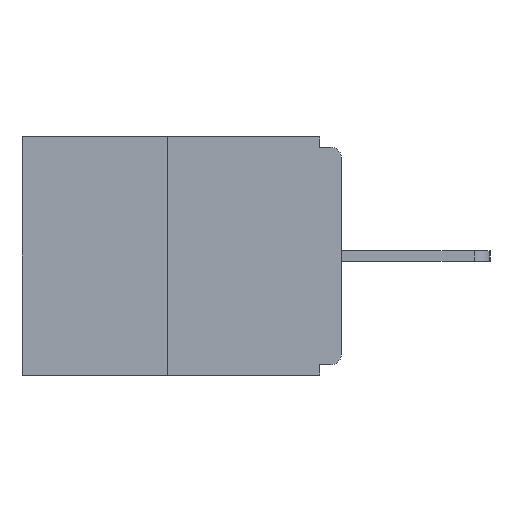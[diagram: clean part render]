
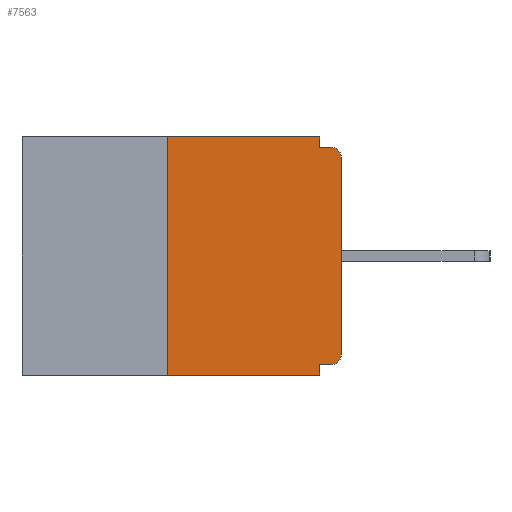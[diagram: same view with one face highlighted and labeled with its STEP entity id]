
A CAD part, left-side view. The second image highlights one B-rep face of the part: STEP entity #7563.
In plain terms, the highlighted planar face has unit normal (-1, 0, 0).
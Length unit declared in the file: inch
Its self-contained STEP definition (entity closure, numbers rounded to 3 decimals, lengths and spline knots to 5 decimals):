
#67 = ORIENTED_EDGE ( 'NONE', *, *, #9139, .T. ) ;
#259 = CARTESIAN_POINT ( 'NONE',  ( 0., 0.46, 0. ) ) ;
#504 = CARTESIAN_POINT ( 'NONE',  ( 0., 0.031, -0.343 ) ) ;
#523 = DIRECTION ( 'NONE',  ( 0., 0., -1. ) ) ;
#675 = ORIENTED_EDGE ( 'NONE', *, *, #9671, .F. ) ;
#726 = PLANE ( 'NONE',  #10815 ) ;
#740 = VECTOR ( 'NONE', #11413, 39.37008 ) ;
#1176 = LINE ( 'NONE', #8990, #740 ) ;
#1315 = DIRECTION ( 'NONE',  ( 0., 0., 1. ) ) ;
#1775 = EDGE_CURVE ( 'NONE', #8409, #5490, #1176, .T. ) ;
#1778 = CARTESIAN_POINT ( 'NONE',  ( 0., 0.46, 0. ) ) ;
#1848 = FACE_OUTER_BOUND ( 'NONE', #5617, .T. ) ;
#1991 = DIRECTION ( 'NONE',  ( 0., -1., 0. ) ) ;
#2332 = CARTESIAN_POINT ( 'NONE',  ( 0., 0.25, -0.343 ) ) ;
#2336 = VERTEX_POINT ( 'NONE', #6966 ) ;
#2339 = EDGE_CURVE ( 'NONE', #11931, #5745, #4573, .T. ) ;
#2678 = DIRECTION ( 'NONE',  ( -1., 0., 0. ) ) ;
#2886 = DIRECTION ( 'NONE',  ( 0., 0., -1. ) ) ;
#3020 = CARTESIAN_POINT ( 'NONE',  ( 0., 0.015, -0.328 ) ) ;
#3303 = CARTESIAN_POINT ( 'NONE',  ( 0., 0., -0.015 ) ) ;
#3915 = CARTESIAN_POINT ( 'NONE',  ( 0., 0.015, -0.03 ) ) ;
#4070 = ORIENTED_EDGE ( 'NONE', *, *, #4232, .T. ) ;
#4172 = LINE ( 'NONE', #8780, #8700 ) ;
#4232 = EDGE_CURVE ( 'NONE', #13693, #10342, #6443, .T. ) ;
#4345 = CARTESIAN_POINT ( 'NONE',  ( 0., 0.031, -0.328 ) ) ;
#4377 = LINE ( 'NONE', #259, #12143 ) ;
#4391 = DIRECTION ( 'NONE',  ( 0., 0., 1. ) ) ;
#4573 = LINE ( 'NONE', #11536, #8085 ) ;
#4588 = VECTOR ( 'NONE', #1315, 39.37008 ) ;
#5240 = VECTOR ( 'NONE', #11384, 39.37008 ) ;
#5322 = CARTESIAN_POINT ( 'NONE',  ( 0., 0.46, -0.343 ) ) ;
#5490 = VERTEX_POINT ( 'NONE', #13238 ) ;
#5492 = EDGE_CURVE ( 'NONE', #5490, #11547, #8824, .T. ) ;
#5617 = EDGE_LOOP ( 'NONE', ( #9534, #675, #4070, #6351, #9223, #13205, #8591, #67, #12000, #12722 ) ) ;
#5745 = VERTEX_POINT ( 'NONE', #4345 ) ;
#5790 = CIRCLE ( 'NONE', #8423, 0.015 ) ;
#6094 = CARTESIAN_POINT ( 'NONE',  ( 0., 0.015, -0.313 ) ) ;
#6312 = LINE ( 'NONE', #7933, #11745 ) ;
#6351 = ORIENTED_EDGE ( 'NONE', *, *, #7503, .F. ) ;
#6443 = LINE ( 'NONE', #5322, #12668 ) ;
#6966 = CARTESIAN_POINT ( 'NONE',  ( 0., 0., -0.313 ) ) ;
#7444 = EDGE_CURVE ( 'NONE', #11931, #2336, #7749, .T. ) ;
#7503 = EDGE_CURVE ( 'NONE', #5745, #10342, #6312, .T. ) ;
#7563 = ADVANCED_FACE ( 'NONE', ( #1848 ), #726, .F. ) ;
#7576 = DIRECTION ( 'NONE',  ( 0., 0., -1. ) ) ;
#7749 = CIRCLE ( 'NONE', #9160, 0.015 ) ;
#7826 = CARTESIAN_POINT ( 'NONE',  ( 0., 0.031, 0. ) ) ;
#7933 = CARTESIAN_POINT ( 'NONE',  ( 0., 0.031, -0.343 ) ) ;
#8085 = VECTOR ( 'NONE', #9257, 39.37008 ) ;
#8397 = CARTESIAN_POINT ( 'NONE',  ( 0., 0., -0.03 ) ) ;
#8409 = VERTEX_POINT ( 'NONE', #7826 ) ;
#8423 = AXIS2_PLACEMENT_3D ( 'NONE', #3915, #12954, #8469 ) ;
#8469 = DIRECTION ( 'NONE',  ( 0., 0., -1. ) ) ;
#8550 = DIRECTION ( 'NONE',  ( 1., 0., 0. ) ) ;
#8591 = ORIENTED_EDGE ( 'NONE', *, *, #8983, .T. ) ;
#8700 = VECTOR ( 'NONE', #4391, 39.37008 ) ;
#8780 = CARTESIAN_POINT ( 'NONE',  ( 0., 0.25, 0. ) ) ;
#8824 = LINE ( 'NONE', #3303, #5240 ) ;
#8914 = CARTESIAN_POINT ( 'NONE',  ( 0., 0.015, -0.015 ) ) ;
#8920 = DIRECTION ( 'NONE',  ( 0., -1., 0. ) ) ;
#8983 = EDGE_CURVE ( 'NONE', #2336, #10373, #11474, .T. ) ;
#8990 = CARTESIAN_POINT ( 'NONE',  ( 0., 0.031, 0. ) ) ;
#9139 = EDGE_CURVE ( 'NONE', #10373, #11547, #5790, .T. ) ;
#9160 = AXIS2_PLACEMENT_3D ( 'NONE', #6094, #2678, #523 ) ;
#9223 = ORIENTED_EDGE ( 'NONE', *, *, #2339, .F. ) ;
#9257 = DIRECTION ( 'NONE',  ( 0., 1., 0. ) ) ;
#9534 = ORIENTED_EDGE ( 'NONE', *, *, #14593, .F. ) ;
#9671 = EDGE_CURVE ( 'NONE', #13693, #14512, #4172, .T. ) ;
#9680 = CARTESIAN_POINT ( 'NONE',  ( 0., 0.25, 0. ) ) ;
#10342 = VERTEX_POINT ( 'NONE', #504 ) ;
#10373 = VERTEX_POINT ( 'NONE', #8397 ) ;
#10815 = AXIS2_PLACEMENT_3D ( 'NONE', #1778, #8550, #2886 ) ;
#11331 = CARTESIAN_POINT ( 'NONE',  ( 0., 0., 0. ) ) ;
#11384 = DIRECTION ( 'NONE',  ( 0., -1., 0. ) ) ;
#11413 = DIRECTION ( 'NONE',  ( 0., 0., -1. ) ) ;
#11474 = LINE ( 'NONE', #11331, #4588 ) ;
#11536 = CARTESIAN_POINT ( 'NONE',  ( 0., 0., -0.328 ) ) ;
#11547 = VERTEX_POINT ( 'NONE', #8914 ) ;
#11745 = VECTOR ( 'NONE', #7576, 39.37008 ) ;
#11931 = VERTEX_POINT ( 'NONE', #3020 ) ;
#12000 = ORIENTED_EDGE ( 'NONE', *, *, #5492, .F. ) ;
#12143 = VECTOR ( 'NONE', #8920, 39.37008 ) ;
#12668 = VECTOR ( 'NONE', #1991, 39.37008 ) ;
#12722 = ORIENTED_EDGE ( 'NONE', *, *, #1775, .F. ) ;
#12954 = DIRECTION ( 'NONE',  ( -1., 0., 0. ) ) ;
#13205 = ORIENTED_EDGE ( 'NONE', *, *, #7444, .T. ) ;
#13238 = CARTESIAN_POINT ( 'NONE',  ( 0., 0.031, -0.015 ) ) ;
#13693 = VERTEX_POINT ( 'NONE', #2332 ) ;
#14512 = VERTEX_POINT ( 'NONE', #9680 ) ;
#14593 = EDGE_CURVE ( 'NONE', #14512, #8409, #4377, .T. ) ;
